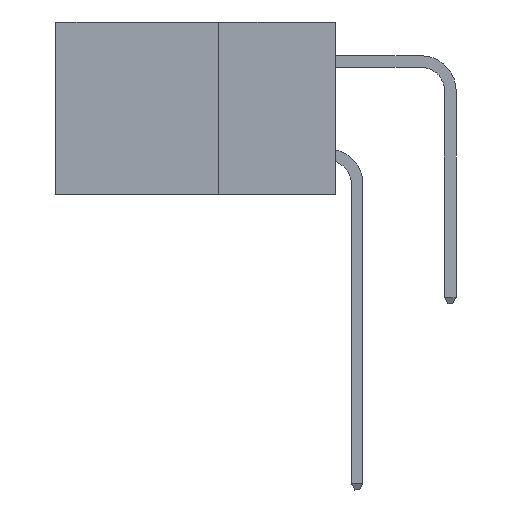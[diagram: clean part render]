
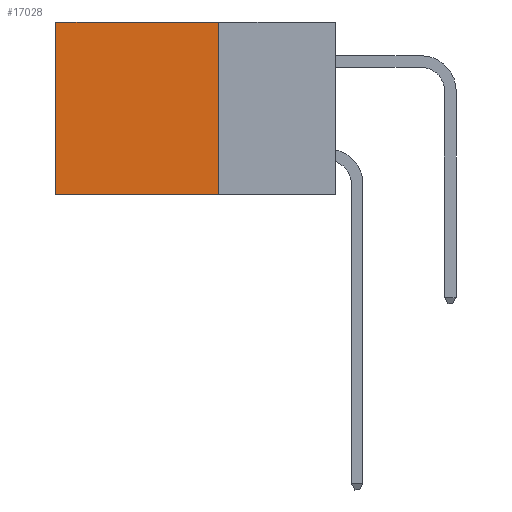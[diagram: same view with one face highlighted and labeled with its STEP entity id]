
A CAD part, left-side view. The second image highlights one B-rep face of the part: STEP entity #17028.
In plain terms, the highlighted planar face has unit normal (-1, 0, 0).
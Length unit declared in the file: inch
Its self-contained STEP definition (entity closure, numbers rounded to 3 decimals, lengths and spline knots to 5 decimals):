
#14 = VERTEX_POINT ( 'NONE', #12750 ) ;
#2553 = LINE ( 'NONE', #17161, #9598 ) ;
#2968 = EDGE_CURVE ( 'NONE', #13187, #4948, #9133, .T. ) ;
#3358 = EDGE_LOOP ( 'NONE', ( #5915, #10504, #5470, #16776 ) ) ;
#3661 = VERTEX_POINT ( 'NONE', #14256 ) ;
#4787 = FACE_OUTER_BOUND ( 'NONE', #3358, .T. ) ;
#4948 = VERTEX_POINT ( 'NONE', #11558 ) ;
#5396 = VECTOR ( 'NONE', #7319, 39.37008 ) ;
#5470 = ORIENTED_EDGE ( 'NONE', *, *, #2968, .F. ) ;
#5870 = VECTOR ( 'NONE', #13899, 39.37008 ) ;
#5880 = VECTOR ( 'NONE', #14283, 39.37008 ) ;
#5886 = AXIS2_PLACEMENT_3D ( 'NONE', #7157, #16385, #8531 ) ;
#5915 = ORIENTED_EDGE ( 'NONE', *, *, #11384, .T. ) ;
#7050 = CARTESIAN_POINT ( 'NONE',  ( 0.2875, 0.25, 0. ) ) ;
#7157 = CARTESIAN_POINT ( 'NONE',  ( 0.2875, 0.25, 0. ) ) ;
#7319 = DIRECTION ( 'NONE',  ( 0., 0., -1. ) ) ;
#8531 = DIRECTION ( 'NONE',  ( 0., 0., -1. ) ) ;
#9050 = CARTESIAN_POINT ( 'NONE',  ( 0.2875, 0.25, 0. ) ) ;
#9133 = LINE ( 'NONE', #13947, #5396 ) ;
#9598 = VECTOR ( 'NONE', #10665, 39.37008 ) ;
#10504 = ORIENTED_EDGE ( 'NONE', *, *, #17605, .F. ) ;
#10665 = DIRECTION ( 'NONE',  ( 0., 0., -1. ) ) ;
#11384 = EDGE_CURVE ( 'NONE', #14, #3661, #2553, .T. ) ;
#11558 = CARTESIAN_POINT ( 'NONE',  ( 0.2875, 0.25, -0.37 ) ) ;
#12247 = EDGE_CURVE ( 'NONE', #13187, #14, #13084, .T. ) ;
#12567 = CARTESIAN_POINT ( 'NONE',  ( 0.2875, 0.25, -0.37 ) ) ;
#12750 = CARTESIAN_POINT ( 'NONE',  ( 0.2875, 0.6, 0. ) ) ;
#13084 = LINE ( 'NONE', #9050, #5880 ) ;
#13187 = VERTEX_POINT ( 'NONE', #7050 ) ;
#13899 = DIRECTION ( 'NONE',  ( 0., 1., 0. ) ) ;
#13903 = LINE ( 'NONE', #12567, #5870 ) ;
#13947 = CARTESIAN_POINT ( 'NONE',  ( 0.2875, 0.25, 0. ) ) ;
#14256 = CARTESIAN_POINT ( 'NONE',  ( 0.2875, 0.6, -0.37 ) ) ;
#14283 = DIRECTION ( 'NONE',  ( 0., 1., 0. ) ) ;
#15084 = PLANE ( 'NONE',  #5886 ) ;
#16385 = DIRECTION ( 'NONE',  ( 1., 0., 0. ) ) ;
#16776 = ORIENTED_EDGE ( 'NONE', *, *, #12247, .T. ) ;
#17028 = ADVANCED_FACE ( 'NONE', ( #4787 ), #15084, .F. ) ;
#17161 = CARTESIAN_POINT ( 'NONE',  ( 0.2875, 0.6, 0. ) ) ;
#17605 = EDGE_CURVE ( 'NONE', #4948, #3661, #13903, .T. ) ;
